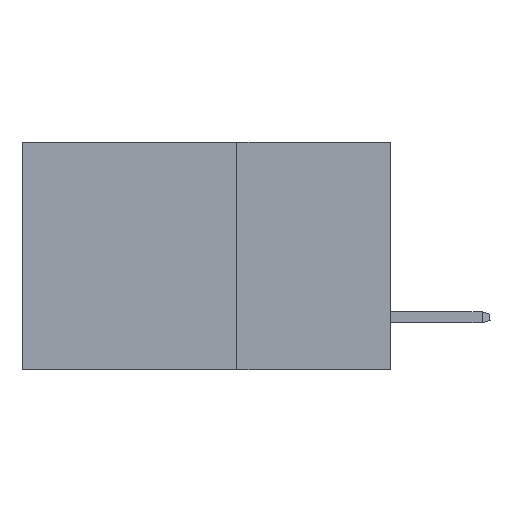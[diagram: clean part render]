
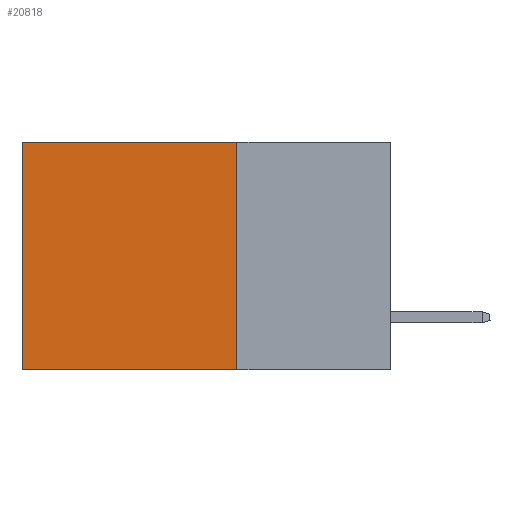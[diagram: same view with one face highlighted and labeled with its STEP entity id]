
A CAD part, left-side view. The second image highlights one B-rep face of the part: STEP entity #20818.
In plain terms, the highlighted planar face has unit normal (-1, 0, 0).
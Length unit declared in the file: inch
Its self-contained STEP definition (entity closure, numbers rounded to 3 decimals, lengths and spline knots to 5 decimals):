
#530 = CARTESIAN_POINT ( 'NONE',  ( 0.2875, 0.25, 0. ) ) ;
#2975 = CARTESIAN_POINT ( 'NONE',  ( 0.2875, 0.25, 0. ) ) ;
#5461 = AXIS2_PLACEMENT_3D ( 'NONE', #2975, #18828, #16143 ) ;
#6450 = PLANE ( 'NONE',  #5461 ) ;
#6647 = CARTESIAN_POINT ( 'NONE',  ( 0.2875, 0.25, -0.37 ) ) ;
#6951 = LINE ( 'NONE', #21965, #16012 ) ;
#9805 = EDGE_CURVE ( 'NONE', #36692, #40655, #13073, .T. ) ;
#12126 = CARTESIAN_POINT ( 'NONE',  ( 0.2875, 0.25, 0. ) ) ;
#13073 = LINE ( 'NONE', #20477, #34155 ) ;
#13492 = DIRECTION ( 'NONE',  ( 0., 0., -1. ) ) ;
#13605 = CARTESIAN_POINT ( 'NONE',  ( 0.2875, 0.25, -0.37 ) ) ;
#14413 = FACE_OUTER_BOUND ( 'NONE', #35282, .T. ) ;
#14736 = ORIENTED_EDGE ( 'NONE', *, *, #9805, .T. ) ;
#14775 = EDGE_CURVE ( 'NONE', #31590, #15103, #27450, .T. ) ;
#15103 = VERTEX_POINT ( 'NONE', #13605 ) ;
#16012 = VECTOR ( 'NONE', #41247, 39.37008 ) ;
#16143 = DIRECTION ( 'NONE',  ( 0., 0., -1. ) ) ;
#16365 = VECTOR ( 'NONE', #13492, 39.37008 ) ;
#18828 = DIRECTION ( 'NONE',  ( 1., 0., 0. ) ) ;
#20477 = CARTESIAN_POINT ( 'NONE',  ( 0.2875, 0.6, 0. ) ) ;
#20818 = ADVANCED_FACE ( 'NONE', ( #14413 ), #6450, .F. ) ;
#21570 = ORIENTED_EDGE ( 'NONE', *, *, #25738, .T. ) ;
#21965 = CARTESIAN_POINT ( 'NONE',  ( 0.2875, 0.25, 0. ) ) ;
#22040 = CARTESIAN_POINT ( 'NONE',  ( 0.2875, 0.6, 0. ) ) ;
#25738 = EDGE_CURVE ( 'NONE', #31590, #36692, #6951, .T. ) ;
#25959 = ORIENTED_EDGE ( 'NONE', *, *, #31071, .F. ) ;
#27450 = LINE ( 'NONE', #530, #16365 ) ;
#29819 = LINE ( 'NONE', #6647, #38772 ) ;
#30586 = ORIENTED_EDGE ( 'NONE', *, *, #14775, .F. ) ;
#31071 = EDGE_CURVE ( 'NONE', #15103, #40655, #29819, .T. ) ;
#31590 = VERTEX_POINT ( 'NONE', #12126 ) ;
#33253 = DIRECTION ( 'NONE',  ( 0., 0., -1. ) ) ;
#34155 = VECTOR ( 'NONE', #33253, 39.37008 ) ;
#35282 = EDGE_LOOP ( 'NONE', ( #14736, #25959, #30586, #21570 ) ) ;
#36612 = CARTESIAN_POINT ( 'NONE',  ( 0.2875, 0.6, -0.37 ) ) ;
#36692 = VERTEX_POINT ( 'NONE', #22040 ) ;
#38748 = DIRECTION ( 'NONE',  ( 0., 1., 0. ) ) ;
#38772 = VECTOR ( 'NONE', #38748, 39.37008 ) ;
#40655 = VERTEX_POINT ( 'NONE', #36612 ) ;
#41247 = DIRECTION ( 'NONE',  ( 0., 1., 0. ) ) ;
